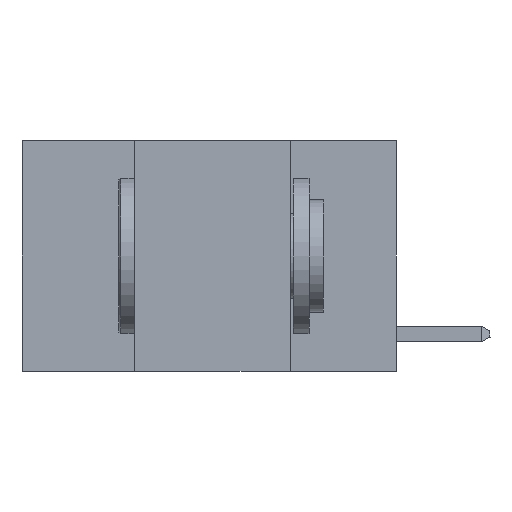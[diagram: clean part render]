
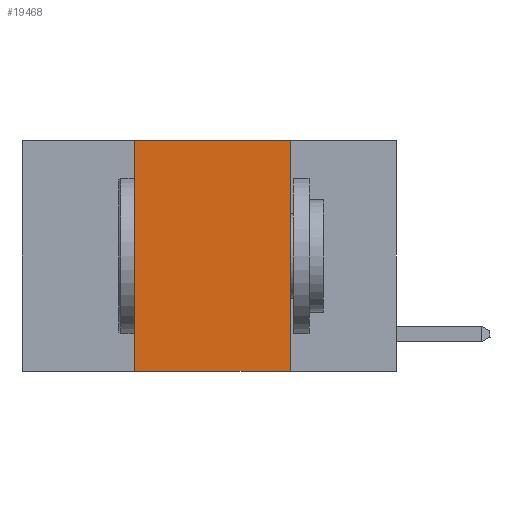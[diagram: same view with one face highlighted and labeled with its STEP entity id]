
A CAD part, left-side view. The second image highlights one B-rep face of the part: STEP entity #19468.
In plain terms, the highlighted planar face has unit normal (-1, 0, 0).
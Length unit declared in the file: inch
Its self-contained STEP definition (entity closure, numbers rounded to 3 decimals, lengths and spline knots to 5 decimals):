
#107 = CARTESIAN_POINT ( 'NONE',  ( 0., 0.42, 0. ) ) ;
#1965 = PLANE ( 'NONE',  #18814 ) ;
#1994 = DIRECTION ( 'NONE',  ( 0., 0., -1. ) ) ;
#2572 = VECTOR ( 'NONE', #20107, 39.37008 ) ;
#3785 = CARTESIAN_POINT ( 'NONE',  ( 0., 0.17, -0.37 ) ) ;
#5982 = ORIENTED_EDGE ( 'NONE', *, *, #12473, .F. ) ;
#6287 = VECTOR ( 'NONE', #24038, 39.37008 ) ;
#6779 = VERTEX_POINT ( 'NONE', #107 ) ;
#7147 = EDGE_CURVE ( 'NONE', #10632, #6779, #22335, .T. ) ;
#7204 = LINE ( 'NONE', #21942, #6287 ) ;
#7516 = CARTESIAN_POINT ( 'NONE',  ( 0., 0.17, 0. ) ) ;
#7540 = CARTESIAN_POINT ( 'NONE',  ( 0., 0.6, -0.37 ) ) ;
#8210 = VECTOR ( 'NONE', #1994, 39.37008 ) ;
#8743 = ORIENTED_EDGE ( 'NONE', *, *, #22187, .F. ) ;
#10632 = VERTEX_POINT ( 'NONE', #13294 ) ;
#10685 = CARTESIAN_POINT ( 'NONE',  ( 0., 0.17, 0. ) ) ;
#11494 = ORIENTED_EDGE ( 'NONE', *, *, #7147, .F. ) ;
#12473 = EDGE_CURVE ( 'NONE', #13305, #12690, #20784, .T. ) ;
#12690 = VERTEX_POINT ( 'NONE', #3785 ) ;
#13294 = CARTESIAN_POINT ( 'NONE',  ( 0., 0.42, -0.37 ) ) ;
#13305 = VERTEX_POINT ( 'NONE', #10685 ) ;
#15091 = DIRECTION ( 'NONE',  ( 0., -1., 0. ) ) ;
#17018 = DIRECTION ( 'NONE',  ( 1., 0., 0. ) ) ;
#18356 = CARTESIAN_POINT ( 'NONE',  ( 0., 0.42, 0. ) ) ;
#18795 = DIRECTION ( 'NONE',  ( 0., 0., -1. ) ) ;
#18814 = AXIS2_PLACEMENT_3D ( 'NONE', #20635, #17018, #18795 ) ;
#18911 = FACE_OUTER_BOUND ( 'NONE', #19669, .T. ) ;
#19468 = ADVANCED_FACE ( 'NONE', ( #18911 ), #1965, .F. ) ;
#19669 = EDGE_LOOP ( 'NONE', ( #5982, #8743, #11494, #22463 ) ) ;
#20107 = DIRECTION ( 'NONE',  ( 0., 0., 1. ) ) ;
#20297 = EDGE_CURVE ( 'NONE', #10632, #12690, #24264, .T. ) ;
#20635 = CARTESIAN_POINT ( 'NONE',  ( 0., 0.6, 0. ) ) ;
#20784 = LINE ( 'NONE', #7516, #8210 ) ;
#21942 = CARTESIAN_POINT ( 'NONE',  ( 0., 0.6, 0. ) ) ;
#22187 = EDGE_CURVE ( 'NONE', #6779, #13305, #7204, .T. ) ;
#22335 = LINE ( 'NONE', #18356, #2572 ) ;
#22463 = ORIENTED_EDGE ( 'NONE', *, *, #20297, .T. ) ;
#24038 = DIRECTION ( 'NONE',  ( 0., -1., 0. ) ) ;
#24264 = LINE ( 'NONE', #7540, #24378 ) ;
#24378 = VECTOR ( 'NONE', #15091, 39.37008 ) ;
